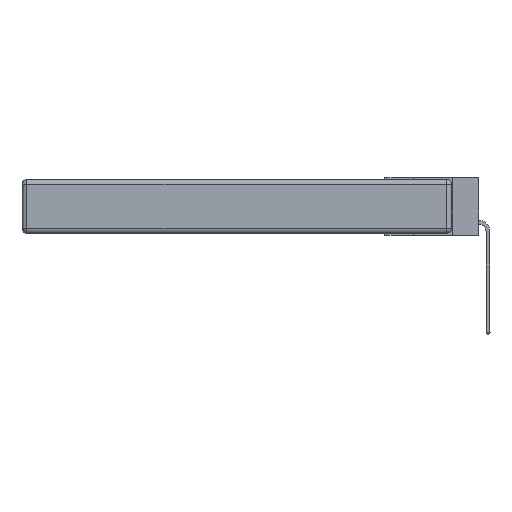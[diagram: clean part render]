
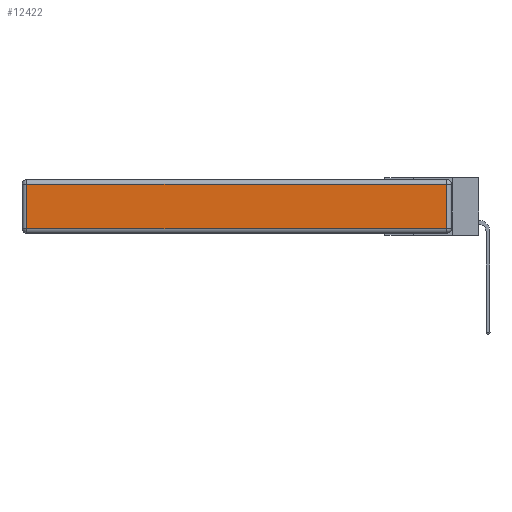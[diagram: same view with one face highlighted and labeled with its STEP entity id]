
A CAD part, left-side view. The second image highlights one B-rep face of the part: STEP entity #12422.
In plain terms, the highlighted planar face has unit normal (-1, 0, 0).
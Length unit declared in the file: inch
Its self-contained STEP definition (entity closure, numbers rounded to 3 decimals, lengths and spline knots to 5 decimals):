
#32 = VERTEX_POINT ( 'NONE', #5024 ) ;
#46 = ORIENTED_EDGE ( 'NONE', *, *, #8022, .T. ) ;
#238 = CARTESIAN_POINT ( 'NONE',  ( 0., 0.03, -0.313 ) ) ;
#380 = CARTESIAN_POINT ( 'NONE',  ( 0., 2.72, -0.313 ) ) ;
#584 = VECTOR ( 'NONE', #2314, 39.37008 ) ;
#620 = VERTEX_POINT ( 'NONE', #14318 ) ;
#746 = VERTEX_POINT ( 'NONE', #238 ) ;
#789 = ORIENTED_EDGE ( 'NONE', *, *, #2119, .T. ) ;
#1309 = VECTOR ( 'NONE', #9830, 39.37008 ) ;
#2073 = FACE_OUTER_BOUND ( 'NONE', #8295, .T. ) ;
#2119 = EDGE_CURVE ( 'NONE', #620, #6353, #11540, .T. ) ;
#2314 = DIRECTION ( 'NONE',  ( 0., 0., 1. ) ) ;
#2345 = EDGE_CURVE ( 'NONE', #32, #620, #8232, .T. ) ;
#3042 = DIRECTION ( 'NONE',  ( -1., 0., 0. ) ) ;
#3136 = CARTESIAN_POINT ( 'NONE',  ( 0., 0., -0.343 ) ) ;
#3399 = ORIENTED_EDGE ( 'NONE', *, *, #2345, .T. ) ;
#3884 = CARTESIAN_POINT ( 'NONE',  ( 0., 2.75, -0.03 ) ) ;
#4286 = DIRECTION ( 'NONE',  ( 0., 0., -1. ) ) ;
#5024 = CARTESIAN_POINT ( 'NONE',  ( 0., 0.03, -0.03 ) ) ;
#5594 = VECTOR ( 'NONE', #4286, 39.37008 ) ;
#5679 = ORIENTED_EDGE ( 'NONE', *, *, #13303, .T. ) ;
#6353 = VERTEX_POINT ( 'NONE', #380 ) ;
#6409 = PLANE ( 'NONE',  #9143 ) ;
#6777 = CARTESIAN_POINT ( 'NONE',  ( 0., 0.03, -0.343 ) ) ;
#8022 = EDGE_CURVE ( 'NONE', #746, #32, #9387, .T. ) ;
#8232 = LINE ( 'NONE', #3884, #8935 ) ;
#8295 = EDGE_LOOP ( 'NONE', ( #5679, #46, #3399, #789 ) ) ;
#8935 = VECTOR ( 'NONE', #11710, 39.37008 ) ;
#9143 = AXIS2_PLACEMENT_3D ( 'NONE', #3136, #3042, #10854 ) ;
#9387 = LINE ( 'NONE', #6777, #584 ) ;
#9785 = CARTESIAN_POINT ( 'NONE',  ( 0., 0., -0.313 ) ) ;
#9830 = DIRECTION ( 'NONE',  ( 0., -1., 0. ) ) ;
#10854 = DIRECTION ( 'NONE',  ( 0., 0., 1. ) ) ;
#11540 = LINE ( 'NONE', #14333, #5594 ) ;
#11710 = DIRECTION ( 'NONE',  ( 0., 1., 0. ) ) ;
#12422 = ADVANCED_FACE ( 'NONE', ( #2073 ), #6409, .T. ) ;
#13303 = EDGE_CURVE ( 'NONE', #6353, #746, #14500, .T. ) ;
#14318 = CARTESIAN_POINT ( 'NONE',  ( 0., 2.72, -0.03 ) ) ;
#14333 = CARTESIAN_POINT ( 'NONE',  ( 0., 2.72, -0.343 ) ) ;
#14500 = LINE ( 'NONE', #9785, #1309 ) ;
